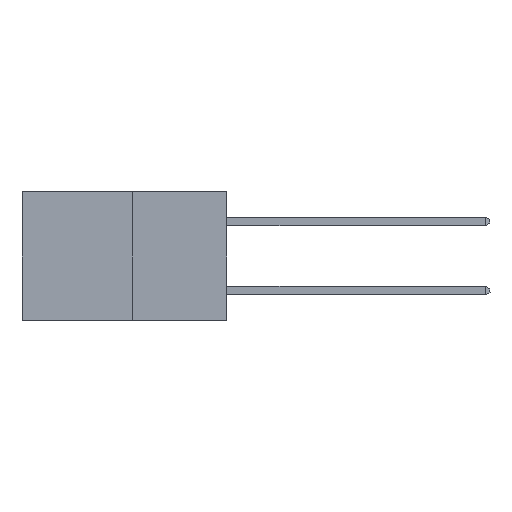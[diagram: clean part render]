
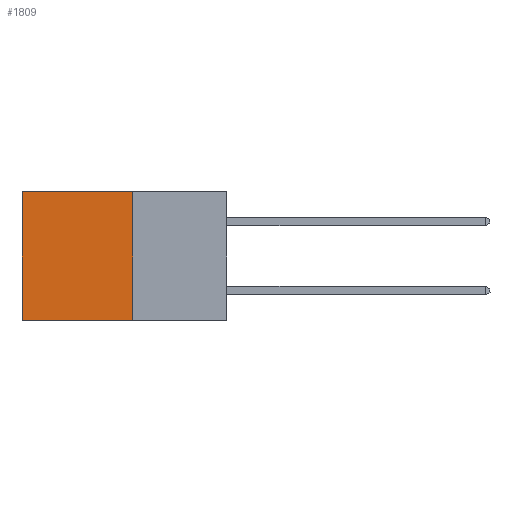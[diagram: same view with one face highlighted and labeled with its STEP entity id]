
A CAD part, left-side view. The second image highlights one B-rep face of the part: STEP entity #1809.
In plain terms, the highlighted planar face has unit normal (-1, 0, 0).
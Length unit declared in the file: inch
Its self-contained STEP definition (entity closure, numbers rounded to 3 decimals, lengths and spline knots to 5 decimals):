
#308 = PLANE ( 'NONE',  #11354 ) ;
#393 = LINE ( 'NONE', #21137, #18081 ) ;
#733 = EDGE_CURVE ( 'NONE', #13189, #1566, #16899, .T. ) ;
#1566 = VERTEX_POINT ( 'NONE', #6701 ) ;
#1809 = ADVANCED_FACE ( 'NONE', ( #8037 ), #308, .F. ) ;
#2701 = VECTOR ( 'NONE', #9207, 39.37008 ) ;
#3642 = EDGE_LOOP ( 'NONE', ( #20708, #9630, #19576, #4328 ) ) ;
#3805 = CARTESIAN_POINT ( 'NONE',  ( 0.277, 0.59, -0.37 ) ) ;
#4043 = EDGE_CURVE ( 'NONE', #11050, #1566, #8458, .T. ) ;
#4328 = ORIENTED_EDGE ( 'NONE', *, *, #14014, .T. ) ;
#5120 = CARTESIAN_POINT ( 'NONE',  ( 0.277, 0.27, -0.37 ) ) ;
#5204 = DIRECTION ( 'NONE',  ( 0., 0., -1. ) ) ;
#6177 = EDGE_CURVE ( 'NONE', #7580, #11050, #20865, .T. ) ;
#6701 = CARTESIAN_POINT ( 'NONE',  ( 0.277, 0.59, -0.37 ) ) ;
#7580 = VERTEX_POINT ( 'NONE', #12140 ) ;
#8037 = FACE_OUTER_BOUND ( 'NONE', #3642, .T. ) ;
#8458 = LINE ( 'NONE', #20290, #21463 ) ;
#9207 = DIRECTION ( 'NONE',  ( 0., 0., -1. ) ) ;
#9630 = ORIENTED_EDGE ( 'NONE', *, *, #4043, .F. ) ;
#11050 = VERTEX_POINT ( 'NONE', #19080 ) ;
#11354 = AXIS2_PLACEMENT_3D ( 'NONE', #21377, #20761, #15612 ) ;
#12140 = CARTESIAN_POINT ( 'NONE',  ( 0.277, 0.27, 0. ) ) ;
#13189 = VERTEX_POINT ( 'NONE', #21975 ) ;
#14014 = EDGE_CURVE ( 'NONE', #7580, #13189, #393, .T. ) ;
#14413 = DIRECTION ( 'NONE',  ( 0., 1., 0. ) ) ;
#15612 = DIRECTION ( 'NONE',  ( 0., 0., -1. ) ) ;
#16403 = VECTOR ( 'NONE', #5204, 39.37008 ) ;
#16899 = LINE ( 'NONE', #3805, #2701 ) ;
#18081 = VECTOR ( 'NONE', #14413, 39.37008 ) ;
#19080 = CARTESIAN_POINT ( 'NONE',  ( 0.277, 0.27, -0.37 ) ) ;
#19191 = DIRECTION ( 'NONE',  ( 0., 1., 0. ) ) ;
#19576 = ORIENTED_EDGE ( 'NONE', *, *, #6177, .F. ) ;
#20290 = CARTESIAN_POINT ( 'NONE',  ( 0.277, 0.27, -0.37 ) ) ;
#20708 = ORIENTED_EDGE ( 'NONE', *, *, #733, .T. ) ;
#20761 = DIRECTION ( 'NONE',  ( 1., 0., 0. ) ) ;
#20865 = LINE ( 'NONE', #5120, #16403 ) ;
#21137 = CARTESIAN_POINT ( 'NONE',  ( 0.277, 0.27, 0. ) ) ;
#21377 = CARTESIAN_POINT ( 'NONE',  ( 0.277, 0.27, -0.37 ) ) ;
#21463 = VECTOR ( 'NONE', #19191, 39.37008 ) ;
#21975 = CARTESIAN_POINT ( 'NONE',  ( 0.277, 0.59, 0. ) ) ;
